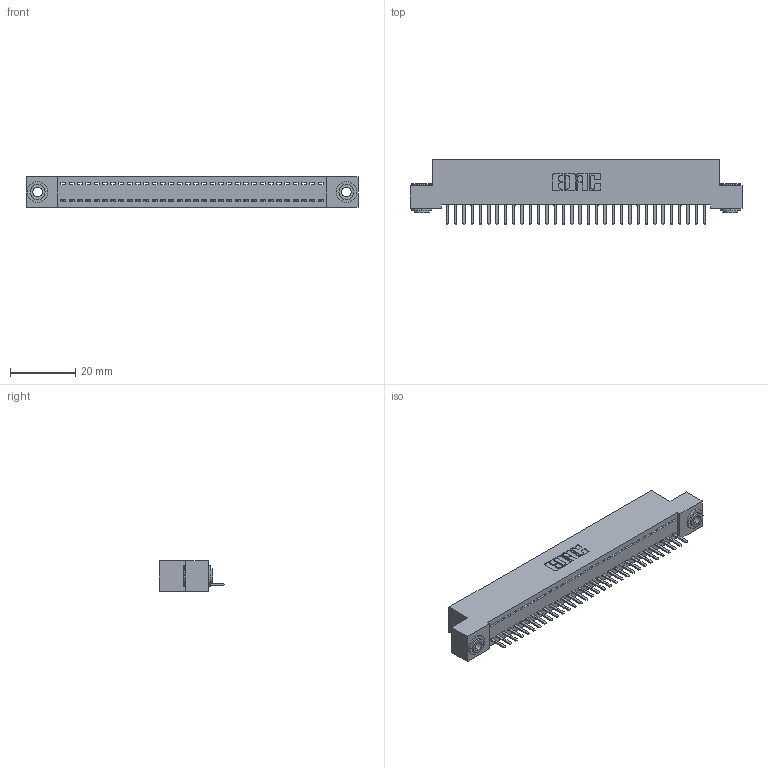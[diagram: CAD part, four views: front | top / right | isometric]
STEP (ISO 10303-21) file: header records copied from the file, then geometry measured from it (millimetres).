
FILE_DESCRIPTION (( 'STEP AP203' ), '1' );
FILE_NAME ('342-032-520-103.STEP', '2019-10-02T06:02:00', ( '' ), ( '' ), 'SwSTEP 2.0', 'SolidWorks 2016', '' );
FILE_SCHEMA (( 'CONFIG_CONTROL_DESIGN' ));
Length unit declared in the file: inch
Products named in the file (4): 342 Part_.156 TH; 345-292-001_345-293-120; 342-250-002_345-250-002-102; 342-032-520-103
Assembly tree (35 placements, depth 2):
  342-032-520-103
    342 Part_.156 TH
    345-292-001_345-293-120  x32
    342-250-002_345-250-002-102  x2
Bounding box: 101.6 x 20.02 x 9.4 mm (x, y, z)
Volume: 8802.2 mm3; surface area: 12670.7 mm2
Topology: 35 solids, 35 shells, 2132 faces, 6263 edges, 4086 vertices
Faces by surface type: plane 1484, cylinder 640, cone 8
Entity records: 21488 total; most frequent: CARTESIAN_POINT 3697, ORIENTED_EDGE 3646, DIRECTION 3161, EDGE_CURVE 1823, VECTOR 1667, LINE 1667, VERTEX_POINT 1210, AXIS2_PLACEMENT_3D 747
